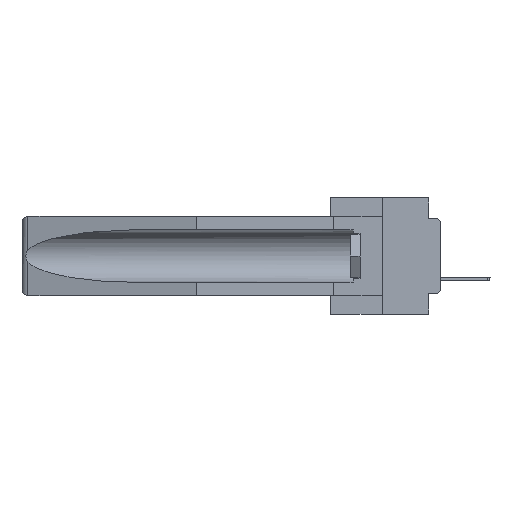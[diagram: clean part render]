
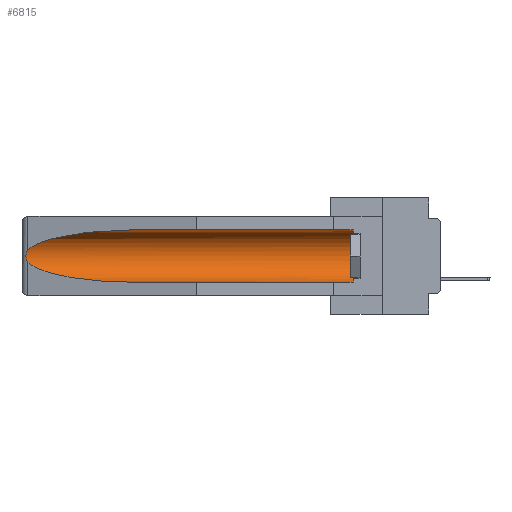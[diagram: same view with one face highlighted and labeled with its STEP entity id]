
A CAD part, left-side view. The second image highlights one B-rep face of the part: STEP entity #6815.
In plain terms, the highlighted cylindrical face has radius 2.857 mm (diameter 5.715 mm), a partial arc.
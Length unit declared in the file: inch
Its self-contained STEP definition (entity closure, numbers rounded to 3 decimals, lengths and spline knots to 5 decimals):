
#143 = VECTOR ( 'NONE', #28502, 39.37008 ) ;
#681 = ORIENTED_EDGE ( 'NONE', *, *, #23541, .F. ) ;
#1073 = LINE ( 'NONE', #3165, #143 ) ;
#1321 = CARTESIAN_POINT ( 'NONE',  ( 0.155, 0.126, -0.284 ) ) ;
#1586 = DIRECTION ( 'NONE',  ( 0., 1., 0. ) ) ;
#1746 = VERTEX_POINT ( 'NONE', #10173 ) ;
#2008 = EDGE_CURVE ( 'NONE', #12094, #1746, #25571, .T. ) ;
#2080 = ORIENTED_EDGE ( 'NONE', *, *, #15931, .T. ) ;
#3127 =( BOUNDED_CURVE ( )  B_SPLINE_CURVE ( 3, ( #28682, #17456, #10672, #19846 ),
 .UNSPECIFIED., .F., .F. ) 
 B_SPLINE_CURVE_WITH_KNOTS ( ( 4, 4 ),
 ( 4.71239, 6.08839 ),
 .UNSPECIFIED. ) 
 CURVE ( )  GEOMETRIC_REPRESENTATION_ITEM ( )  RATIONAL_B_SPLINE_CURVE ( ( 1., 0.848, 0.848, 1. ) ) 
 REPRESENTATION_ITEM ( '' )  );
#3165 = CARTESIAN_POINT ( 'NONE',  ( 0.155, -0.30754, -0.284 ) ) ;
#3299 = CARTESIAN_POINT ( 'NONE',  ( 0.26537, 1.52718, -0.14972 ) ) ;
#3343 = CARTESIAN_POINT ( 'NONE',  ( 0.26537, 1.52718, -0.14972 ) ) ;
#3446 = CARTESIAN_POINT ( 'NONE',  ( 0.26655, 1.53094, -0.18657 ) ) ;
#3979 = CYLINDRICAL_SURFACE ( 'NONE', #21928, 0.1125 ) ;
#4058 = AXIS2_PLACEMENT_3D ( 'NONE', #22978, #18478, #9157 ) ;
#4572 = ORIENTED_EDGE ( 'NONE', *, *, #2008, .T. ) ;
#5803 = VERTEX_POINT ( 'NONE', #3343 ) ;
#5962 = EDGE_CURVE ( 'NONE', #1746, #5803, #3127, .T. ) ;
#6148 = CARTESIAN_POINT ( 'NONE',  ( 0.26597, 1.5296, -0.19026 ) ) ;
#6521 = FACE_OUTER_BOUND ( 'NONE', #24972, .T. ) ;
#6815 = ADVANCED_FACE ( 'NONE', ( #6521 ), #3979, .F. ) ;
#8379 = CARTESIAN_POINT ( 'NONE',  ( 0.26597, 1.52961, -0.15275 ) ) ;
#9157 = DIRECTION ( 'NONE',  ( 0., 0., 1. ) ) ;
#9506 = VERTEX_POINT ( 'NONE', #27422 ) ;
#10173 = CARTESIAN_POINT ( 'NONE',  ( 0.155, 1.07973, -0.059 ) ) ;
#10274 = ORIENTED_EDGE ( 'NONE', *, *, #17123, .T. ) ;
#10672 = CARTESIAN_POINT ( 'NONE',  ( 0.25451, 1.48313, -0.09465 ) ) ;
#12073 = DIRECTION ( 'NONE',  ( 0., 1., 0. ) ) ;
#12094 = VERTEX_POINT ( 'NONE', #25830 ) ;
#12611 = CARTESIAN_POINT ( 'NONE',  ( 0.2675, 1.53308, -0.17534 ) ) ;
#13090 = CARTESIAN_POINT ( 'NONE',  ( 0.25451, 1.48313, -0.24835 ) ) ;
#14608 = CIRCLE ( 'NONE', #4058, 0.1125 ) ;
#15315 = CARTESIAN_POINT ( 'NONE',  ( 0.26537, 1.52718, -0.19328 ) ) ;
#15931 = EDGE_CURVE ( 'NONE', #25110, #12094, #14608, .T. ) ;
#16284 = B_SPLINE_CURVE_WITH_KNOTS ( 'NONE', 3,
 ( #3299, #8379, #17713, #26682, #26827, #12611, #26241, #3446, #6148, #15315 ),
 .UNSPECIFIED., .F., .F.,
 ( 4, 2, 2, 2, 4 ),
 ( 0., 0.00029, 0.00058, 0.00087, 0.00117 ),
 .UNSPECIFIED. ) ;
#17123 = EDGE_CURVE ( 'NONE', #9506, #21523, #26863, .T. ) ;
#17456 = CARTESIAN_POINT ( 'NONE',  ( 0.21114, 1.30732, -0.059 ) ) ;
#17713 = CARTESIAN_POINT ( 'NONE',  ( 0.26654, 1.53092, -0.15636 ) ) ;
#18478 = DIRECTION ( 'NONE',  ( 0., -1., 0. ) ) ;
#18896 = EDGE_CURVE ( 'NONE', #5803, #9506, #16284, .T. ) ;
#19828 = CARTESIAN_POINT ( 'NONE',  ( 0.155, 1.07973, -0.284 ) ) ;
#19846 = CARTESIAN_POINT ( 'NONE',  ( 0.26537, 1.52718, -0.14972 ) ) ;
#21523 = VERTEX_POINT ( 'NONE', #24680 ) ;
#21560 = VECTOR ( 'NONE', #12073, 39.37008 ) ;
#21928 = AXIS2_PLACEMENT_3D ( 'NONE', #22439, #1586, #26767 ) ;
#22439 = CARTESIAN_POINT ( 'NONE',  ( 0.155, -0.30754, -0.1715 ) ) ;
#22978 = CARTESIAN_POINT ( 'NONE',  ( 0.155, 0.126, -0.1715 ) ) ;
#23541 = EDGE_CURVE ( 'NONE', #25110, #21523, #1073, .T. ) ;
#24336 = CARTESIAN_POINT ( 'NONE',  ( 0.21114, 1.30732, -0.284 ) ) ;
#24680 = CARTESIAN_POINT ( 'NONE',  ( 0.155, 1.07973, -0.284 ) ) ;
#24972 = EDGE_LOOP ( 'NONE', ( #27642, #28879, #10274, #681, #2080, #4572 ) ) ;
#25110 = VERTEX_POINT ( 'NONE', #1321 ) ;
#25571 = LINE ( 'NONE', #28260, #21560 ) ;
#25830 = CARTESIAN_POINT ( 'NONE',  ( 0.155, 0.126, -0.059 ) ) ;
#26241 = CARTESIAN_POINT ( 'NONE',  ( 0.2673, 1.53269, -0.17917 ) ) ;
#26561 = CARTESIAN_POINT ( 'NONE',  ( 0.26537, 1.52718, -0.19328 ) ) ;
#26682 = CARTESIAN_POINT ( 'NONE',  ( 0.2673, 1.5327, -0.16383 ) ) ;
#26767 = DIRECTION ( 'NONE',  ( 0., 0., 1. ) ) ;
#26827 = CARTESIAN_POINT ( 'NONE',  ( 0.2675, 1.53308, -0.16763 ) ) ;
#26863 =( BOUNDED_CURVE ( )  B_SPLINE_CURVE ( 3, ( #26561, #13090, #24336, #19828 ),
 .UNSPECIFIED., .F., .F. ) 
 B_SPLINE_CURVE_WITH_KNOTS ( ( 4, 4 ),
 ( 0.1948, 1.5708 ),
 .UNSPECIFIED. ) 
 CURVE ( )  GEOMETRIC_REPRESENTATION_ITEM ( )  RATIONAL_B_SPLINE_CURVE ( ( 1., 0.848, 0.848, 1. ) ) 
 REPRESENTATION_ITEM ( '' )  );
#27422 = CARTESIAN_POINT ( 'NONE',  ( 0.26537, 1.52718, -0.19328 ) ) ;
#27642 = ORIENTED_EDGE ( 'NONE', *, *, #5962, .T. ) ;
#28260 = CARTESIAN_POINT ( 'NONE',  ( 0.155, -0.30754, -0.059 ) ) ;
#28502 = DIRECTION ( 'NONE',  ( 0., 1., 0. ) ) ;
#28682 = CARTESIAN_POINT ( 'NONE',  ( 0.155, 1.07973, -0.059 ) ) ;
#28879 = ORIENTED_EDGE ( 'NONE', *, *, #18896, .T. ) ;
